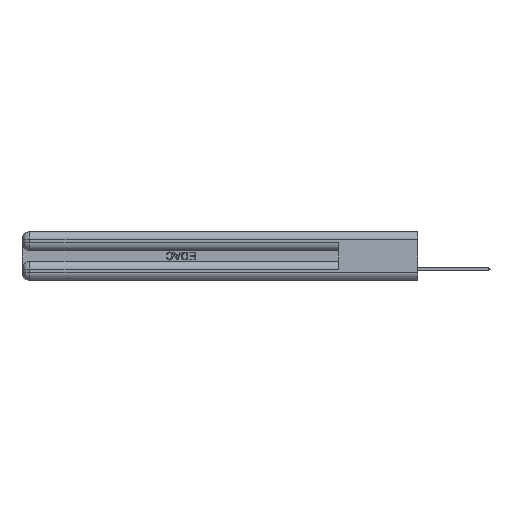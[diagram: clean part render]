
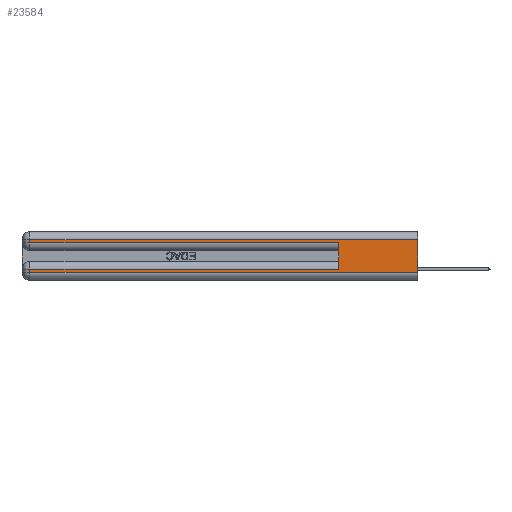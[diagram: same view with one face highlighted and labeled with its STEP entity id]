
A CAD part, left-side view. The second image highlights one B-rep face of the part: STEP entity #23584.
In plain terms, the highlighted planar face has unit normal (-1, 0, 0).
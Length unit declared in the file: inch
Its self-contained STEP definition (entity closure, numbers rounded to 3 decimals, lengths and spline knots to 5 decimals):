
#48 = ORIENTED_EDGE ( 'NONE', *, *, #46280, .T. ) ;
#326 = CARTESIAN_POINT ( 'NONE',  ( 0., 0., 0.06 ) ) ;
#969 = LINE ( 'NONE', #43048, #27513 ) ;
#2063 = FACE_OUTER_BOUND ( 'NONE', #33158, .T. ) ;
#3803 = CARTESIAN_POINT ( 'NONE',  ( 0., 0., 0.085 ) ) ;
#4177 = VERTEX_POINT ( 'NONE', #9253 ) ;
#4199 = PLANE ( 'NONE',  #33543 ) ;
#4500 = DIRECTION ( 'NONE',  ( 1., 0., 0. ) ) ;
#4665 = CARTESIAN_POINT ( 'NONE',  ( 0., 0., 0.285 ) ) ;
#4837 = DIRECTION ( 'NONE',  ( 0., -1., 0. ) ) ;
#5470 = EDGE_CURVE ( 'NONE', #39223, #40590, #40607, .T. ) ;
#7605 = ORIENTED_EDGE ( 'NONE', *, *, #10965, .T. ) ;
#8339 = LINE ( 'NONE', #12650, #46252 ) ;
#9253 = CARTESIAN_POINT ( 'NONE',  ( 0., 2.94, 0.31 ) ) ;
#9831 = VECTOR ( 'NONE', #42996, 39.37008 ) ;
#10872 = DIRECTION ( 'NONE',  ( 0., 1., 0. ) ) ;
#10965 = EDGE_CURVE ( 'NONE', #4177, #39223, #34919, .T. ) ;
#11151 = ORIENTED_EDGE ( 'NONE', *, *, #5470, .T. ) ;
#12090 = CARTESIAN_POINT ( 'NONE',  ( 0., 2.94, 0.285 ) ) ;
#12650 = CARTESIAN_POINT ( 'NONE',  ( 0., 0.6, 0.145 ) ) ;
#12858 = VECTOR ( 'NONE', #4837, 39.37008 ) ;
#14627 = EDGE_CURVE ( 'NONE', #40200, #16353, #35550, .T. ) ;
#14940 = CARTESIAN_POINT ( 'NONE',  ( 0., 2.94, 0.06 ) ) ;
#15628 = EDGE_CURVE ( 'NONE', #40200, #40590, #8339, .T. ) ;
#16332 = CARTESIAN_POINT ( 'NONE',  ( 0., 0.6, 0.285 ) ) ;
#16353 = VERTEX_POINT ( 'NONE', #47907 ) ;
#17295 = CARTESIAN_POINT ( 'NONE',  ( 0., 0.6, 0.085 ) ) ;
#18400 = LINE ( 'NONE', #42831, #9831 ) ;
#18423 = CARTESIAN_POINT ( 'NONE',  ( 0., 2.94, 0.37 ) ) ;
#19370 = VERTEX_POINT ( 'NONE', #19896 ) ;
#19896 = CARTESIAN_POINT ( 'NONE',  ( 0., 0., 0.31 ) ) ;
#20294 = DIRECTION ( 'NONE',  ( 0., 0., 1. ) ) ;
#23584 = ADVANCED_FACE ( 'NONE', ( #2063 ), #4199, .F. ) ;
#23631 = CARTESIAN_POINT ( 'NONE',  ( 0., 0., 0.37 ) ) ;
#24188 = ORIENTED_EDGE ( 'NONE', *, *, #15628, .F. ) ;
#27513 = VECTOR ( 'NONE', #31451, 39.37008 ) ;
#27912 = EDGE_CURVE ( 'NONE', #19370, #43913, #42117, .T. ) ;
#28808 = VECTOR ( 'NONE', #42129, 39.37008 ) ;
#29820 = ORIENTED_EDGE ( 'NONE', *, *, #46220, .T. ) ;
#31127 = ORIENTED_EDGE ( 'NONE', *, *, #39316, .T. ) ;
#31175 = DIRECTION ( 'NONE',  ( 0., 0., -1. ) ) ;
#31188 = LINE ( 'NONE', #326, #28808 ) ;
#31451 = DIRECTION ( 'NONE',  ( 0., 1., 0. ) ) ;
#33158 = EDGE_LOOP ( 'NONE', ( #34903, #48, #7605, #11151, #24188, #48329, #31127, #29820 ) ) ;
#33543 = AXIS2_PLACEMENT_3D ( 'NONE', #23631, #4500, #31175 ) ;
#34339 = VECTOR ( 'NONE', #47401, 39.37008 ) ;
#34903 = ORIENTED_EDGE ( 'NONE', *, *, #27912, .F. ) ;
#34919 = LINE ( 'NONE', #18423, #45763 ) ;
#35550 = LINE ( 'NONE', #3803, #37484 ) ;
#35687 = CARTESIAN_POINT ( 'NONE',  ( 0., 0., 0.37 ) ) ;
#37484 = VECTOR ( 'NONE', #10872, 39.37008 ) ;
#39223 = VERTEX_POINT ( 'NONE', #12090 ) ;
#39316 = EDGE_CURVE ( 'NONE', #16353, #42371, #18400, .T. ) ;
#39961 = CARTESIAN_POINT ( 'NONE',  ( 0., 0., 0.06 ) ) ;
#40200 = VERTEX_POINT ( 'NONE', #17295 ) ;
#40590 = VERTEX_POINT ( 'NONE', #16332 ) ;
#40607 = LINE ( 'NONE', #4665, #12858 ) ;
#42117 = LINE ( 'NONE', #35687, #34339 ) ;
#42129 = DIRECTION ( 'NONE',  ( 0., -1., 0. ) ) ;
#42371 = VERTEX_POINT ( 'NONE', #14940 ) ;
#42831 = CARTESIAN_POINT ( 'NONE',  ( 0., 2.94, 0.37 ) ) ;
#42996 = DIRECTION ( 'NONE',  ( 0., 0., -1. ) ) ;
#43048 = CARTESIAN_POINT ( 'NONE',  ( 0., 0., 0.31 ) ) ;
#43913 = VERTEX_POINT ( 'NONE', #39961 ) ;
#45763 = VECTOR ( 'NONE', #48750, 39.37008 ) ;
#46220 = EDGE_CURVE ( 'NONE', #42371, #43913, #31188, .T. ) ;
#46252 = VECTOR ( 'NONE', #20294, 39.37008 ) ;
#46280 = EDGE_CURVE ( 'NONE', #19370, #4177, #969, .T. ) ;
#47401 = DIRECTION ( 'NONE',  ( 0., 0., -1. ) ) ;
#47907 = CARTESIAN_POINT ( 'NONE',  ( 0., 2.94, 0.085 ) ) ;
#48329 = ORIENTED_EDGE ( 'NONE', *, *, #14627, .T. ) ;
#48750 = DIRECTION ( 'NONE',  ( 0., 0., -1. ) ) ;
